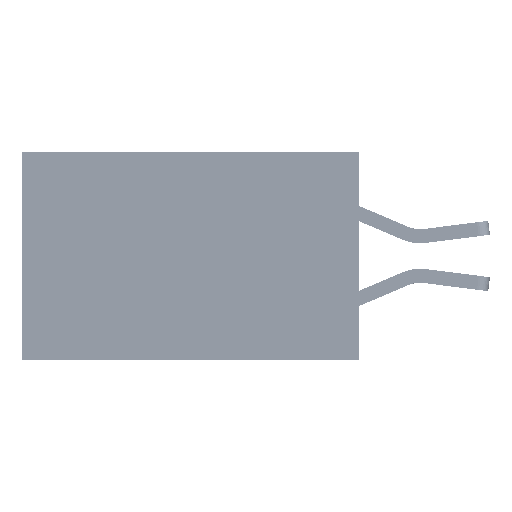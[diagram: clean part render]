
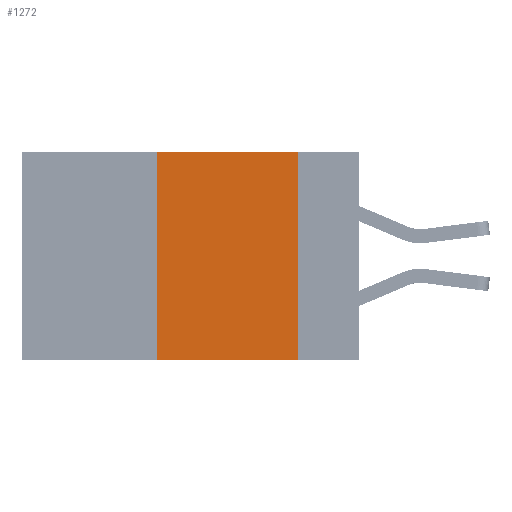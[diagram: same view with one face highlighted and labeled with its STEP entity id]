
A CAD part, left-side view. The second image highlights one B-rep face of the part: STEP entity #1272.
In plain terms, the highlighted planar face has unit normal (-1, 0, 0).
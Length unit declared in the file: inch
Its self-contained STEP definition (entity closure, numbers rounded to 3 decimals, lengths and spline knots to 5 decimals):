
#1272 = ADVANCED_FACE ( 'NONE', ( #6153 ), #29752, .F. ) ;
#4516 = CARTESIAN_POINT ( 'NONE',  ( 0., 0.11, 0. ) ) ;
#6153 = FACE_OUTER_BOUND ( 'NONE', #10546, .T. ) ;
#8958 = AXIS2_PLACEMENT_3D ( 'NONE', #22147, #41128, #33736 ) ;
#9659 = VERTEX_POINT ( 'NONE', #4516 ) ;
#10546 = EDGE_LOOP ( 'NONE', ( #42066, #18926, #19935, #35034 ) ) ;
#11108 = VECTOR ( 'NONE', #13255, 39.37008 ) ;
#13255 = DIRECTION ( 'NONE',  ( 0., -1., 0. ) ) ;
#13457 = CARTESIAN_POINT ( 'NONE',  ( 0., 0.11, 0. ) ) ;
#15038 = VERTEX_POINT ( 'NONE', #48025 ) ;
#17349 = LINE ( 'NONE', #31496, #22633 ) ;
#17913 = DIRECTION ( 'NONE',  ( 0., 0., -1. ) ) ;
#18926 = ORIENTED_EDGE ( 'NONE', *, *, #30593, .F. ) ;
#19935 = ORIENTED_EDGE ( 'NONE', *, *, #20759, .F. ) ;
#20759 = EDGE_CURVE ( 'NONE', #30726, #15038, #24373, .T. ) ;
#20887 = VERTEX_POINT ( 'NONE', #46845 ) ;
#21375 = LINE ( 'NONE', #13457, #28480 ) ;
#22147 = CARTESIAN_POINT ( 'NONE',  ( 0., 0.6, 0. ) ) ;
#22633 = VECTOR ( 'NONE', #24032, 39.37008 ) ;
#24032 = DIRECTION ( 'NONE',  ( 0., -1., 0. ) ) ;
#24373 = LINE ( 'NONE', #45851, #36795 ) ;
#28480 = VECTOR ( 'NONE', #17913, 39.37008 ) ;
#29462 = LINE ( 'NONE', #43945, #11108 ) ;
#29752 = PLANE ( 'NONE',  #8958 ) ;
#30593 = EDGE_CURVE ( 'NONE', #15038, #9659, #17349, .T. ) ;
#30726 = VERTEX_POINT ( 'NONE', #40215 ) ;
#31496 = CARTESIAN_POINT ( 'NONE',  ( 0., 0.6, 0. ) ) ;
#33736 = DIRECTION ( 'NONE',  ( 0., 0., -1. ) ) ;
#35034 = ORIENTED_EDGE ( 'NONE', *, *, #47953, .T. ) ;
#36795 = VECTOR ( 'NONE', #38444, 39.37008 ) ;
#37512 = EDGE_CURVE ( 'NONE', #9659, #20887, #21375, .T. ) ;
#38444 = DIRECTION ( 'NONE',  ( 0., 0., 1. ) ) ;
#40215 = CARTESIAN_POINT ( 'NONE',  ( 0., 0.36, -0.37 ) ) ;
#41128 = DIRECTION ( 'NONE',  ( 1., 0., 0. ) ) ;
#42066 = ORIENTED_EDGE ( 'NONE', *, *, #37512, .F. ) ;
#43945 = CARTESIAN_POINT ( 'NONE',  ( 0., 0.6, -0.37 ) ) ;
#45851 = CARTESIAN_POINT ( 'NONE',  ( 0., 0.36, 0. ) ) ;
#46845 = CARTESIAN_POINT ( 'NONE',  ( 0., 0.11, -0.37 ) ) ;
#47953 = EDGE_CURVE ( 'NONE', #30726, #20887, #29462, .T. ) ;
#48025 = CARTESIAN_POINT ( 'NONE',  ( 0., 0.36, 0. ) ) ;
